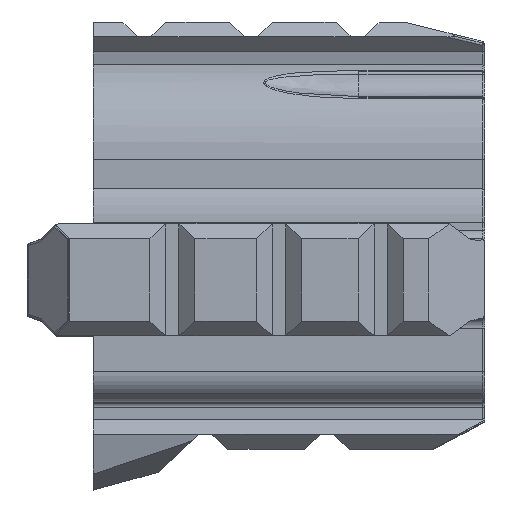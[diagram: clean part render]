
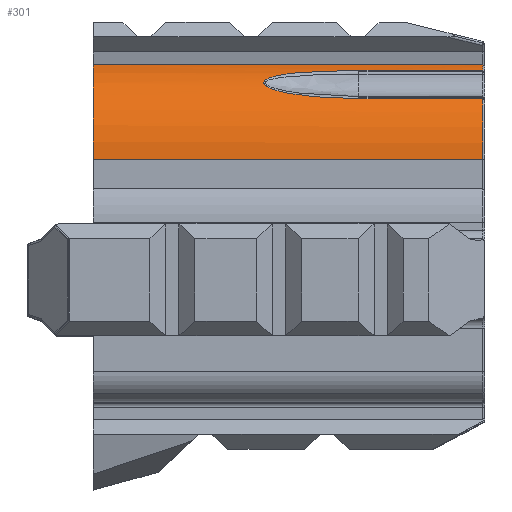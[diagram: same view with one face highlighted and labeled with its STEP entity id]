
A CAD part, top view. The second image highlights one B-rep face of the part: STEP entity #301.
In plain terms, the highlighted cylindrical face has radius 20.1 mm (diameter 40.2 mm), a partial arc.
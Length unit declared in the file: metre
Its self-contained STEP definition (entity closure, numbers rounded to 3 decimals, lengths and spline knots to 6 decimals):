
#301=ADVANCED_FACE('0:150',(#993),#994,.T.);
#993=FACE_OUTER_BOUND('',#3013,.T.);
#994=CYLINDRICAL_SURFACE('',#3014,0.0201);
#3013=EDGE_LOOP('',(#5726,#5727,#5728,#5729,#5730,#5731,#5732,#5733,#5734));
#3014=AXIS2_PLACEMENT_3D('',#5735,#5736,#5737);
#5726=ORIENTED_EDGE('',*,*,#7887,.F.);
#5727=ORIENTED_EDGE('',*,*,#7319,.F.);
#5728=ORIENTED_EDGE('',*,*,#7901,.F.);
#5729=ORIENTED_EDGE('',*,*,#7315,.F.);
#5730=ORIENTED_EDGE('',*,*,#7891,.F.);
#5731=ORIENTED_EDGE('',*,*,#7625,.T.);
#5732=ORIENTED_EDGE('',*,*,#7646,.F.);
#5733=ORIENTED_EDGE('',*,*,#7610,.T.);
#5734=ORIENTED_EDGE('',*,*,#7895,.F.);
#5735=CARTESIAN_POINT('',(-0.012072,0.047361,0.001));
#5736=DIRECTION('',(-1.0,0.0,-0.0));
#5737=DIRECTION('',(0.0,0.0,-1.0));
#7315=EDGE_CURVE('0:1401',#8613,#8615,#8616,.T.);
#7319=EDGE_CURVE('0:1392',#8621,#8623,#8624,.T.);
#7610=EDGE_CURVE('0:1413',#9147,#9145,#9148,.T.);
#7625=EDGE_CURVE('8:3469',#9165,#9171,#9173,.T.);
#7646=EDGE_CURVE('0:1410',#9147,#9171,#9205,.T.);
#7887=EDGE_CURVE('0:1332',#8623,#9536,#9540,.T.);
#7891=EDGE_CURVE('0:1356',#9165,#8613,#9545,.T.);
#7895=EDGE_CURVE('0:1380',#9536,#9145,#9549,.T.);
#7901=EDGE_CURVE('0:1407',#8615,#8621,#9557,.T.);
#8613=VERTEX_POINT('NONE',#10561);
#8615=VERTEX_POINT('NONE',#10563);
#8616=LINE('',#10564,#10565);
#8621=VERTEX_POINT('NONE',#10576);
#8623=VERTEX_POINT('NONE',#10581);
#8624=LINE('',#10582,#10583);
#9145=VERTEX_POINT('NONE',#11577);
#9147=VERTEX_POINT('NONE',#11580);
#9148=CIRCLE('',#11581,0.0201);
#9165=VERTEX_POINT('',#11604);
#9171=VERTEX_POINT('',#11614);
#9173=ELLIPSE('',#11617,0.028426,0.0201);
#9205=LINE('',#11665,#11666);
#9536=VERTEX_POINT('NONE',#12553);
#9540=CIRCLE('',#12560,0.0201);
#9545=CIRCLE('',#12566,0.0201);
#9549=LINE('',#12573,#12574);
#9557=B_SPLINE_CURVE_WITH_KNOTS('',3,(#12601,#12602,#12603,#12604,#12605,#12606,#12607,#12608,#12609,#12610,#12611,#12612,#12613,#12614,#12615,#12616,#12617,#12618,#12619),.UNSPECIFIED.,.F.,.F.,(4,1,1,1,1,1,1,1,1,1,1,1,1,1,1,1,4),(0.0,0.142857,0.214286,0.25,0.285714,0.357143,0.428571,0.452381,0.47619,0.488095,0.5,0.52381,0.571429,0.595238,0.619048,0.714286,1.0),.UNSPECIFIED.);
#10561=CARTESIAN_POINT('',(0.0883,0.064924,0.010776));
#10563=CARTESIAN_POINT('',(0.06396,0.064924,0.010776));
#10564=CARTESIAN_POINT('',(0.190555,0.064924,0.010776));
#10565=VECTOR('',#13761,1.0);
#10576=CARTESIAN_POINT('',(0.06396,0.059295,0.017174));
#10581=CARTESIAN_POINT('',(0.0883,0.059295,0.017174));
#10582=CARTESIAN_POINT('',(0.190555,0.059295,0.017174));
#10583=VECTOR('',#13763,1.0);
#11577=CARTESIAN_POINT('',(0.011678,0.047361,0.0211));
#11580=CARTESIAN_POINT('',(0.011678,0.065991,0.008545));
#11581=AXIS2_PLACEMENT_3D('',#14315,#14316,#14317);
#11604=CARTESIAN_POINT('',(0.0883,0.065999,0.008527));
#11614=CARTESIAN_POINT('',(0.08828,0.065991,0.008545));
#11617=AXIS2_PLACEMENT_3D('',#14339,#14340,#14341);
#11665=CARTESIAN_POINT('',(-0.012072,0.065991,0.008545));
#11666=VECTOR('',#14371,1.0);
#12553=CARTESIAN_POINT('',(0.0883,0.047361,0.0211));
#12560=AXIS2_PLACEMENT_3D('',#14770,#14771,#14772);
#12566=AXIS2_PLACEMENT_3D('',#14780,#14781,#14782);
#12573=CARTESIAN_POINT('',(-0.012072,0.047361,0.0211));
#12574=VECTOR('',#14786,1.0);
#12601=CARTESIAN_POINT('',(0.06396,0.064924,0.010776));
#12602=CARTESIAN_POINT('',(0.062068,0.064924,0.010776));
#12603=CARTESIAN_POINT('',(0.059228,0.06488,0.010855));
#12604=CARTESIAN_POINT('',(0.055931,0.064737,0.011106));
#12605=CARTESIAN_POINT('',(0.054049,0.064619,0.011305));
#12606=CARTESIAN_POINT('',(0.052173,0.064474,0.011546));
#12607=CARTESIAN_POINT('',(0.049862,0.064227,0.01194));
#12608=CARTESIAN_POINT('',(0.047724,0.06386,0.01249));
#12609=CARTESIAN_POINT('',(0.046315,0.063423,0.013087));
#12610=CARTESIAN_POINT('',(0.045675,0.063116,0.013486));
#12611=CARTESIAN_POINT('',(0.045302,0.062776,0.013902));
#12612=CARTESIAN_POINT('',(0.045137,0.062339,0.014412));
#12613=CARTESIAN_POINT('',(0.045726,0.061611,0.015192));
#12614=CARTESIAN_POINT('',(0.046878,0.061167,0.01561));
#12615=CARTESIAN_POINT('',(0.048041,0.060807,0.015942));
#12616=CARTESIAN_POINT('',(0.049861,0.060363,0.016333));
#12617=CARTESIAN_POINT('',(0.05512,0.059523,0.01702));
#12618=CARTESIAN_POINT('',(0.060176,0.059295,0.017174));
#12619=CARTESIAN_POINT('',(0.06396,0.059295,0.017174));
#13761=DIRECTION('',(-1.0,0.0,0.));
#13763=DIRECTION('',(1.0,0.0,0.));
#14315=CARTESIAN_POINT('',(0.011678,0.047361,0.001));
#14316=DIRECTION('',(1.0,0.,0.0));
#14317=DIRECTION('',(0.0,0.0,-1.0));
#14339=CARTESIAN_POINT('',(0.091573,0.047361,0.001));
#14340=DIRECTION('',(0.707,-0.154,0.69));
#14341=DIRECTION('',(0.707,0.154,-0.69));
#14371=DIRECTION('',(1.0,0.0,0.));
#14770=CARTESIAN_POINT('',(0.0883,0.047361,0.001));
#14771=DIRECTION('',(1.0,0.,0.0));
#14772=DIRECTION('',(0.0,0.0,1.0));
#14780=CARTESIAN_POINT('',(0.0883,0.047361,0.001));
#14781=DIRECTION('',(1.0,0.,0.0));
#14782=DIRECTION('',(0.0,0.0,1.0));
#14786=DIRECTION('',(-1.0,0.0,0.));
